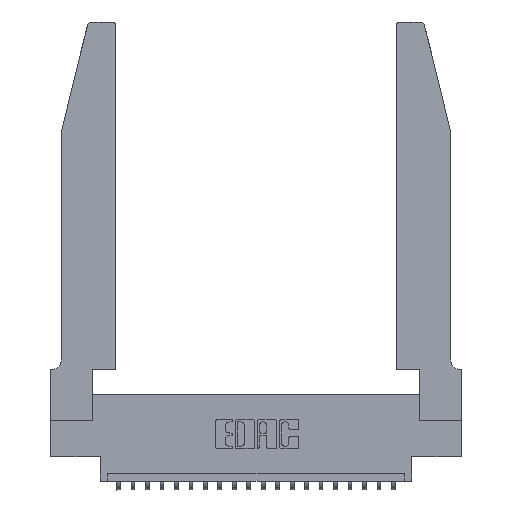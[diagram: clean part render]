
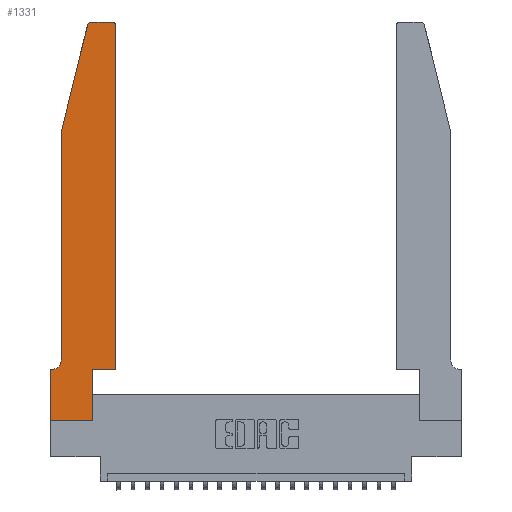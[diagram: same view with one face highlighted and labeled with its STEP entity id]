
A CAD part, top view. The second image highlights one B-rep face of the part: STEP entity #1331.
In plain terms, the highlighted planar face has unit normal (0, 0, 1).
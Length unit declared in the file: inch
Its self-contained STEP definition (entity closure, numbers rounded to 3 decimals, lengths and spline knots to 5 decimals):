
#110 = VERTEX_POINT ( 'NONE', #4078 ) ;
#1331 = ADVANCED_FACE ( 'NONE', ( #1732 ), #16806, .T. ) ;
#1371 = CARTESIAN_POINT ( 'NONE',  ( 0., 0., 0.37 ) ) ;
#1432 = VERTEX_POINT ( 'NONE', #10154 ) ;
#1591 = LINE ( 'NONE', #18300, #2128 ) ;
#1732 = FACE_OUTER_BOUND ( 'NONE', #18801, .T. ) ;
#1810 = DIRECTION ( 'NONE',  ( -1., 0., 0. ) ) ;
#1883 = DIRECTION ( 'NONE',  ( 0., 0., 1. ) ) ;
#1954 = VERTEX_POINT ( 'NONE', #17174 ) ;
#2128 = VECTOR ( 'NONE', #6080, 39.37008 ) ;
#2446 = LINE ( 'NONE', #8111, #6585 ) ;
#2854 = CIRCLE ( 'NONE', #5237, 0.07 ) ;
#2868 = DIRECTION ( 'NONE',  ( 1., 0., 0. ) ) ;
#3645 = DIRECTION ( 'NONE',  ( 1., 0., 0. ) ) ;
#3821 = ORIENTED_EDGE ( 'NONE', *, *, #16141, .T. ) ;
#3963 = AXIS2_PLACEMENT_3D ( 'NONE', #20358, #13473, #9682 ) ;
#3976 = ORIENTED_EDGE ( 'NONE', *, *, #22490, .T. ) ;
#4010 = CARTESIAN_POINT ( 'NONE',  ( 0.0755, 0.35, 0.37 ) ) ;
#4078 = CARTESIAN_POINT ( 'NONE',  ( 0.284, 2.75, 0.37 ) ) ;
#4771 = LINE ( 'NONE', #19831, #19233 ) ;
#4888 = ORIENTED_EDGE ( 'NONE', *, *, #14674, .T. ) ;
#5175 = AXIS2_PLACEMENT_3D ( 'NONE', #10420, #12043, #11961 ) ;
#5237 = AXIS2_PLACEMENT_3D ( 'NONE', #13990, #7234, #17562 ) ;
#5557 = DIRECTION ( 'NONE',  ( -1., 0., 0. ) ) ;
#5787 = VECTOR ( 'NONE', #15866, 39.37008 ) ;
#6080 = DIRECTION ( 'NONE',  ( 0., -1., 0. ) ) ;
#6142 = EDGE_CURVE ( 'NONE', #1954, #110, #22493, .T. ) ;
#6192 = VERTEX_POINT ( 'NONE', #1371 ) ;
#6420 = ORIENTED_EDGE ( 'NONE', *, *, #22334, .T. ) ;
#6585 = VECTOR ( 'NONE', #11654, 39.37008 ) ;
#6772 = CARTESIAN_POINT ( 'NONE',  ( 0.25487, 2.72718, 0.37 ) ) ;
#7234 = DIRECTION ( 'NONE',  ( 0., 0., -1. ) ) ;
#7280 = CARTESIAN_POINT ( 'NONE',  ( 0., 0.35, 0.37 ) ) ;
#7415 = CARTESIAN_POINT ( 'NONE',  ( 0.0755, 0.42, 0.37 ) ) ;
#7765 = CARTESIAN_POINT ( 'NONE',  ( 0.4505, 0.35, 0.37 ) ) ;
#7816 = CIRCLE ( 'NONE', #5175, 0.03 ) ;
#8111 = CARTESIAN_POINT ( 'NONE',  ( 0.2865, 0.35, 0.37 ) ) ;
#8125 = ORIENTED_EDGE ( 'NONE', *, *, #6142, .T. ) ;
#8190 = VERTEX_POINT ( 'NONE', #9887 ) ;
#8792 = LINE ( 'NONE', #10987, #18792 ) ;
#9682 = DIRECTION ( 'NONE',  ( 1., 0., 0. ) ) ;
#9887 = CARTESIAN_POINT ( 'NONE',  ( 0.0055, 0.35, 0.37 ) ) ;
#10154 = CARTESIAN_POINT ( 'NONE',  ( 0.0755, 2., 0.37 ) ) ;
#10237 = CARTESIAN_POINT ( 'NONE',  ( 0.2605, 2.75, 0.37 ) ) ;
#10420 = CARTESIAN_POINT ( 'NONE',  ( 0.4205, 2.72, 0.37 ) ) ;
#10517 = LINE ( 'NONE', #12214, #5787 ) ;
#10699 = CARTESIAN_POINT ( 'NONE',  ( 0.284, 2.72, 0.37 ) ) ;
#10987 = CARTESIAN_POINT ( 'NONE',  ( 0., 0., 0.37 ) ) ;
#11318 = VECTOR ( 'NONE', #13802, 39.37008 ) ;
#11338 = CIRCLE ( 'NONE', #20005, 0.03 ) ;
#11615 = ORIENTED_EDGE ( 'NONE', *, *, #21202, .T. ) ;
#11624 = VERTEX_POINT ( 'NONE', #7415 ) ;
#11654 = DIRECTION ( 'NONE',  ( 0., 1., 0. ) ) ;
#11897 = VERTEX_POINT ( 'NONE', #14126 ) ;
#11961 = DIRECTION ( 'NONE',  ( 1., 0., 0. ) ) ;
#12043 = DIRECTION ( 'NONE',  ( 0., 0., 1. ) ) ;
#12214 = CARTESIAN_POINT ( 'NONE',  ( 0.4505, 0.35, 0.37 ) ) ;
#12401 = LINE ( 'NONE', #4010, #12940 ) ;
#12684 = DIRECTION ( 'NONE',  ( 1., 0., 0. ) ) ;
#12940 = VECTOR ( 'NONE', #5557, 39.37008 ) ;
#13410 = VERTEX_POINT ( 'NONE', #7765 ) ;
#13473 = DIRECTION ( 'NONE',  ( 0., 0., 1. ) ) ;
#13557 = EDGE_CURVE ( 'NONE', #110, #18161, #11338, .T. ) ;
#13709 = CARTESIAN_POINT ( 'NONE',  ( 0.0755, 2., 0.37 ) ) ;
#13802 = DIRECTION ( 'NONE',  ( -0.239, -0.971, 0. ) ) ;
#13990 = CARTESIAN_POINT ( 'NONE',  ( 0.0055, 0.42, 0.37 ) ) ;
#14126 = CARTESIAN_POINT ( 'NONE',  ( 0.4505, 2.72, 0.37 ) ) ;
#14129 = VECTOR ( 'NONE', #15323, 39.37008 ) ;
#14230 = EDGE_CURVE ( 'NONE', #18161, #1432, #16040, .T. ) ;
#14327 = CARTESIAN_POINT ( 'NONE',  ( 0.2865, 0., 0.37 ) ) ;
#14351 = ORIENTED_EDGE ( 'NONE', *, *, #13557, .T. ) ;
#14674 = EDGE_CURVE ( 'NONE', #16498, #20400, #2446, .T. ) ;
#15323 = DIRECTION ( 'NONE',  ( 0., -1., 0. ) ) ;
#15419 = CARTESIAN_POINT ( 'NONE',  ( 0.0755, 2., 0.37 ) ) ;
#15866 = DIRECTION ( 'NONE',  ( 0., 1., 0. ) ) ;
#15882 = CARTESIAN_POINT ( 'NONE',  ( 0.2865, 0.35, 0.37 ) ) ;
#16040 = LINE ( 'NONE', #15419, #11318 ) ;
#16141 = EDGE_CURVE ( 'NONE', #11897, #1954, #7816, .T. ) ;
#16387 = ORIENTED_EDGE ( 'NONE', *, *, #21045, .T. ) ;
#16498 = VERTEX_POINT ( 'NONE', #14327 ) ;
#16806 = PLANE ( 'NONE',  #3963 ) ;
#16862 = EDGE_CURVE ( 'NONE', #1432, #11624, #17748, .T. ) ;
#17090 = ORIENTED_EDGE ( 'NONE', *, *, #14230, .T. ) ;
#17174 = CARTESIAN_POINT ( 'NONE',  ( 0.4205, 2.75, 0.37 ) ) ;
#17208 = EDGE_CURVE ( 'NONE', #13410, #11897, #10517, .T. ) ;
#17545 = ORIENTED_EDGE ( 'NONE', *, *, #16862, .T. ) ;
#17562 = DIRECTION ( 'NONE',  ( -1., 0., 0. ) ) ;
#17748 = LINE ( 'NONE', #13709, #14129 ) ;
#17864 = ORIENTED_EDGE ( 'NONE', *, *, #22262, .T. ) ;
#17899 = VERTEX_POINT ( 'NONE', #7280 ) ;
#18161 = VERTEX_POINT ( 'NONE', #6772 ) ;
#18177 = ORIENTED_EDGE ( 'NONE', *, *, #17208, .T. ) ;
#18300 = CARTESIAN_POINT ( 'NONE',  ( 0., 0., 0.37 ) ) ;
#18792 = VECTOR ( 'NONE', #12684, 39.37008 ) ;
#18801 = EDGE_LOOP ( 'NONE', ( #8125, #14351, #17090, #17545, #16387, #17864, #3976, #6420, #4888, #11615, #18177, #3821 ) ) ;
#18867 = VECTOR ( 'NONE', #1810, 39.37008 ) ;
#19233 = VECTOR ( 'NONE', #2868, 39.37008 ) ;
#19831 = CARTESIAN_POINT ( 'NONE',  ( 0.4505, 0.35, 0.37 ) ) ;
#20005 = AXIS2_PLACEMENT_3D ( 'NONE', #10699, #1883, #3645 ) ;
#20358 = CARTESIAN_POINT ( 'NONE',  ( 0., 0.35, 0.37 ) ) ;
#20400 = VERTEX_POINT ( 'NONE', #15882 ) ;
#21045 = EDGE_CURVE ( 'NONE', #11624, #8190, #2854, .T. ) ;
#21202 = EDGE_CURVE ( 'NONE', #20400, #13410, #4771, .T. ) ;
#22262 = EDGE_CURVE ( 'NONE', #8190, #17899, #12401, .T. ) ;
#22334 = EDGE_CURVE ( 'NONE', #6192, #16498, #8792, .T. ) ;
#22490 = EDGE_CURVE ( 'NONE', #17899, #6192, #1591, .T. ) ;
#22493 = LINE ( 'NONE', #10237, #18867 ) ;
